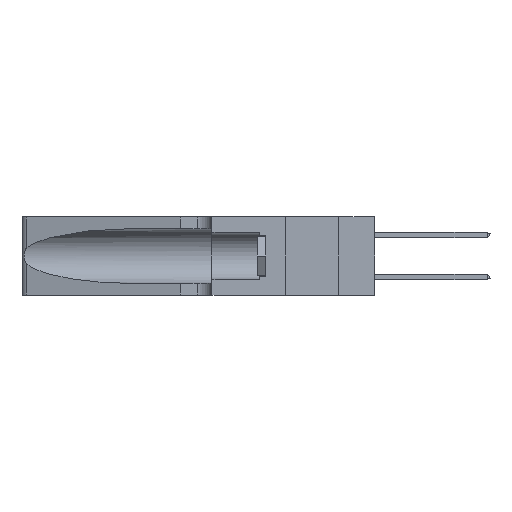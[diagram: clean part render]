
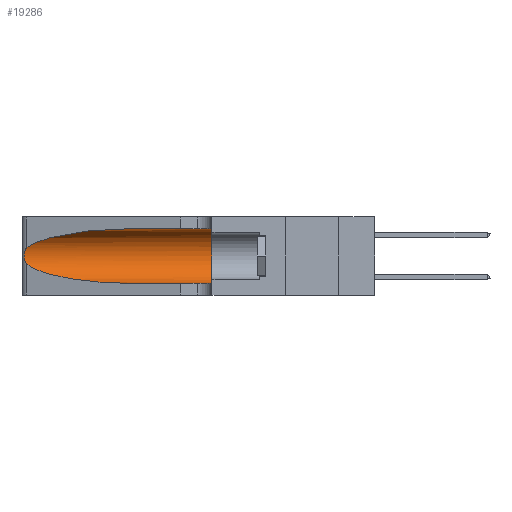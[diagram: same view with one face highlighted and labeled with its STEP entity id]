
A CAD part, left-side view. The second image highlights one B-rep face of the part: STEP entity #19286.
In plain terms, the highlighted cylindrical face has radius 3.308 mm (diameter 6.617 mm), a partial arc.
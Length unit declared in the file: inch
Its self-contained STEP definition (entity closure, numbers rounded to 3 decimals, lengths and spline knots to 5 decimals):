
#461 = CARTESIAN_POINT ( 'NONE',  ( 0.2373, 1.15595, 0.28018 ) ) ;
#1453 = CARTESIAN_POINT ( 'NONE',  ( 0.26075, 1.23896, 0.19203 ) ) ;
#1691 = CARTESIAN_POINT ( 'NONE',  ( 0.25487, 1.22718, 0.22369 ) ) ;
#1864 = CARTESIAN_POINT ( 'NONE',  ( 0.1305, 1.61858, 0.31525 ) ) ;
#2263 = CIRCLE ( 'NONE', #6890, 0.13025 ) ;
#2555 = VERTEX_POINT ( 'NONE', #7412 ) ;
#2604 = CYLINDRICAL_SURFACE ( 'NONE', #10522, 0.13025 ) ;
#2655 = B_SPLINE_CURVE_WITH_KNOTS ( 'NONE', 3,
 ( #4932, #3186, #20287, #10115, #21970, #11817, #1453, #13546, #3259, #15237, #4998, #16948, #6743, #18660 ),
 .UNSPECIFIED., .F., .F.,
 ( 4, 2, 2, 2, 2, 2, 4 ),
 ( 0., 0.00027, 0.00053, 0.00107, 0.0016, 0.00187, 0.00214 ),
 .UNSPECIFIED. ) ;
#2904 = DIRECTION ( 'NONE',  ( 0., -1., 0. ) ) ;
#2950 = VERTEX_POINT ( 'NONE', #16038 ) ;
#3152 = EDGE_LOOP ( 'NONE', ( #9393, #10435, #5284, #10983, #19274, #19003 ) ) ;
#3171 = FACE_OUTER_BOUND ( 'NONE', #3152, .T. ) ;
#3186 = CARTESIAN_POINT ( 'NONE',  ( 0.25555, 1.22994, 0.2215 ) ) ;
#3235 =( BOUNDED_CURVE ( )  B_SPLINE_CURVE ( 3, ( #19375, #21065, #461, #12627 ),
 .UNSPECIFIED., .F., .F. ) 
 B_SPLINE_CURVE_WITH_KNOTS ( ( 4, 4 ),
 ( 1.5708, 2.84003 ),
 .UNSPECIFIED. ) 
 CURVE ( )  GEOMETRIC_REPRESENTATION_ITEM ( )  RATIONAL_B_SPLINE_CURVE ( ( 1., 0.87, 0.87, 1. ) ) 
 REPRESENTATION_ITEM ( '' )  );
#3259 = CARTESIAN_POINT ( 'NONE',  ( 0.26017, 1.23833, 0.17102 ) ) ;
#3653 = DIRECTION ( 'NONE',  ( 0., -1., 0. ) ) ;
#4871 = LINE ( 'NONE', #16615, #13976 ) ;
#4932 = CARTESIAN_POINT ( 'NONE',  ( 0.25487, 1.22718, 0.22369 ) ) ;
#4998 = CARTESIAN_POINT ( 'NONE',  ( 0.25789, 1.23486, 0.15765 ) ) ;
#5028 =( BOUNDED_CURVE ( )  B_SPLINE_CURVE ( 3, ( #16080, #19492, #9308, #21170 ),
 .UNSPECIFIED., .F., .T. ) 
 B_SPLINE_CURVE_WITH_KNOTS ( ( 4, 4 ),
 ( 3.44316, 4.71239 ),
 .UNSPECIFIED. ) 
 CURVE ( )  GEOMETRIC_REPRESENTATION_ITEM ( )  RATIONAL_B_SPLINE_CURVE ( ( 1., 0.87, 0.87, 1. ) ) 
 REPRESENTATION_ITEM ( '' )  );
#5284 = ORIENTED_EDGE ( 'NONE', *, *, #5462, .T. ) ;
#5462 = EDGE_CURVE ( 'NONE', #2555, #17694, #5028, .T. ) ;
#6743 = CARTESIAN_POINT ( 'NONE',  ( 0.25555, 1.22993, 0.14849 ) ) ;
#6890 = AXIS2_PLACEMENT_3D ( 'NONE', #7732, #19644, #9472 ) ;
#6933 = EDGE_CURVE ( 'NONE', #8765, #21130, #13687, .T. ) ;
#7412 = CARTESIAN_POINT ( 'NONE',  ( 0.25487, 1.22718, 0.14631 ) ) ;
#7587 = DIRECTION ( 'NONE',  ( 0., -1., 0. ) ) ;
#7732 = CARTESIAN_POINT ( 'NONE',  ( 0.1305, 0.35, 0.185 ) ) ;
#8692 = EDGE_CURVE ( 'NONE', #17694, #2950, #4871, .T. ) ;
#8765 = VERTEX_POINT ( 'NONE', #9991 ) ;
#9308 = CARTESIAN_POINT ( 'NONE',  ( 0.18966, 0.96281, 0.05475 ) ) ;
#9393 = ORIENTED_EDGE ( 'NONE', *, *, #14323, .T. ) ;
#9433 = CARTESIAN_POINT ( 'NONE',  ( 0.1305, 0.72297, 0.05475 ) ) ;
#9472 = DIRECTION ( 'NONE',  ( 0., 0., 1. ) ) ;
#9991 = CARTESIAN_POINT ( 'NONE',  ( 0.1305, 0.72297, 0.31525 ) ) ;
#10115 = CARTESIAN_POINT ( 'NONE',  ( 0.25787, 1.23484, 0.2124 ) ) ;
#10142 = VERTEX_POINT ( 'NONE', #1691 ) ;
#10435 = ORIENTED_EDGE ( 'NONE', *, *, #15385, .T. ) ;
#10522 = AXIS2_PLACEMENT_3D ( 'NONE', #17798, #7587, #19507 ) ;
#10892 = CARTESIAN_POINT ( 'NONE',  ( 0.1305, 0.35, 0.31525 ) ) ;
#10983 = ORIENTED_EDGE ( 'NONE', *, *, #8692, .T. ) ;
#11817 = CARTESIAN_POINT ( 'NONE',  ( 0.26018, 1.23835, 0.19895 ) ) ;
#12627 = CARTESIAN_POINT ( 'NONE',  ( 0.25487, 1.22718, 0.22369 ) ) ;
#13546 = CARTESIAN_POINT ( 'NONE',  ( 0.26075, 1.23896, 0.178 ) ) ;
#13687 = LINE ( 'NONE', #1864, #22136 ) ;
#13976 = VECTOR ( 'NONE', #2904, 39.37008 ) ;
#14323 = EDGE_CURVE ( 'NONE', #8765, #10142, #3235, .T. ) ;
#15037 = EDGE_CURVE ( 'NONE', #21130, #2950, #2263, .T. ) ;
#15237 = CARTESIAN_POINT ( 'NONE',  ( 0.25856, 1.23593, 0.16098 ) ) ;
#15385 = EDGE_CURVE ( 'NONE', #10142, #2555, #2655, .T. ) ;
#16038 = CARTESIAN_POINT ( 'NONE',  ( 0.1305, 0.35, 0.05475 ) ) ;
#16080 = CARTESIAN_POINT ( 'NONE',  ( 0.25487, 1.22718, 0.14631 ) ) ;
#16615 = CARTESIAN_POINT ( 'NONE',  ( 0.1305, 1.61858, 0.05475 ) ) ;
#16948 = CARTESIAN_POINT ( 'NONE',  ( 0.25639, 1.23186, 0.15144 ) ) ;
#17694 = VERTEX_POINT ( 'NONE', #9433 ) ;
#17798 = CARTESIAN_POINT ( 'NONE',  ( 0.1305, 1.61858, 0.185 ) ) ;
#18660 = CARTESIAN_POINT ( 'NONE',  ( 0.25487, 1.22718, 0.14631 ) ) ;
#19003 = ORIENTED_EDGE ( 'NONE', *, *, #6933, .F. ) ;
#19274 = ORIENTED_EDGE ( 'NONE', *, *, #15037, .F. ) ;
#19286 = ADVANCED_FACE ( 'NONE', ( #3171 ), #2604, .F. ) ;
#19375 = CARTESIAN_POINT ( 'NONE',  ( 0.1305, 0.72297, 0.31525 ) ) ;
#19492 = CARTESIAN_POINT ( 'NONE',  ( 0.2373, 1.15595, 0.08982 ) ) ;
#19507 = DIRECTION ( 'NONE',  ( 0., 0., -1. ) ) ;
#19644 = DIRECTION ( 'NONE',  ( 0., 1., 0. ) ) ;
#20287 = CARTESIAN_POINT ( 'NONE',  ( 0.25639, 1.23184, 0.21858 ) ) ;
#21065 = CARTESIAN_POINT ( 'NONE',  ( 0.18966, 0.96281, 0.31525 ) ) ;
#21130 = VERTEX_POINT ( 'NONE', #10892 ) ;
#21170 = CARTESIAN_POINT ( 'NONE',  ( 0.1305, 0.72297, 0.05475 ) ) ;
#21970 = CARTESIAN_POINT ( 'NONE',  ( 0.25854, 1.2359, 0.20912 ) ) ;
#22136 = VECTOR ( 'NONE', #3653, 39.37008 ) ;
